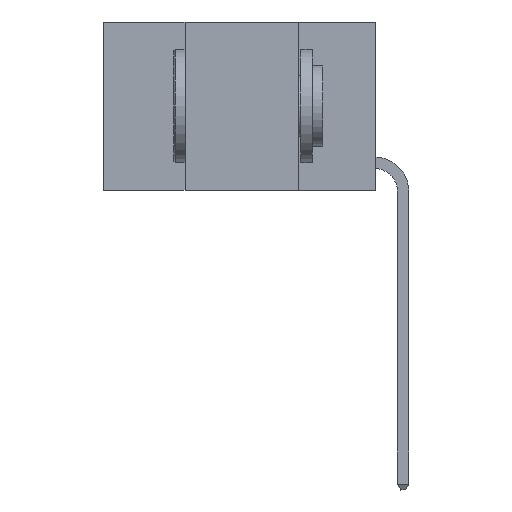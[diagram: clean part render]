
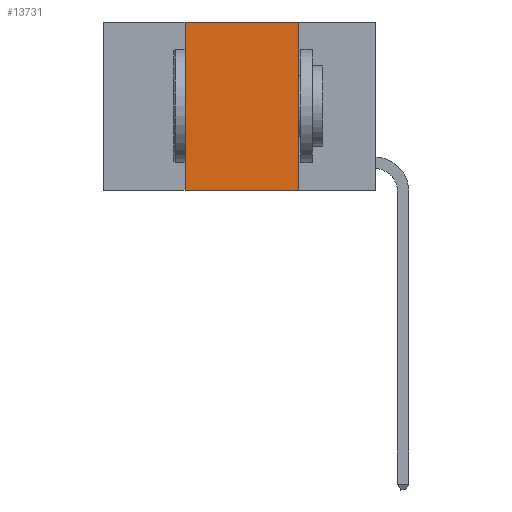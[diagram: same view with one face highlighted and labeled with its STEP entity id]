
A CAD part, left-side view. The second image highlights one B-rep face of the part: STEP entity #13731.
In plain terms, the highlighted planar face has unit normal (-1, 0, 0).
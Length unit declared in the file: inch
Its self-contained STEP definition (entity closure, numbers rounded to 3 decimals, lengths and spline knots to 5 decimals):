
#467 = VERTEX_POINT ( 'NONE', #2920 ) ;
#873 = VECTOR ( 'NONE', #13140, 39.37008 ) ;
#2773 = VERTEX_POINT ( 'NONE', #14449 ) ;
#2920 = CARTESIAN_POINT ( 'NONE',  ( 0., 0.17, 0. ) ) ;
#3199 = EDGE_CURVE ( 'NONE', #2773, #18432, #14423, .T. ) ;
#5081 = ORIENTED_EDGE ( 'NONE', *, *, #13745, .F. ) ;
#6326 = CARTESIAN_POINT ( 'NONE',  ( 0., 0.6, 0. ) ) ;
#6336 = VERTEX_POINT ( 'NONE', #13965 ) ;
#6507 = CARTESIAN_POINT ( 'NONE',  ( 0., 0.42, 0. ) ) ;
#7191 = EDGE_CURVE ( 'NONE', #467, #18432, #13002, .T. ) ;
#8119 = FACE_OUTER_BOUND ( 'NONE', #16934, .T. ) ;
#8319 = VECTOR ( 'NONE', #13219, 39.37008 ) ;
#9045 = CARTESIAN_POINT ( 'NONE',  ( 0., 0.17, -0.37 ) ) ;
#9633 = DIRECTION ( 'NONE',  ( 0., -1., 0. ) ) ;
#9694 = DIRECTION ( 'NONE',  ( 1., 0., 0. ) ) ;
#9911 = EDGE_CURVE ( 'NONE', #2773, #6336, #11960, .T. ) ;
#10307 = VECTOR ( 'NONE', #18775, 39.37008 ) ;
#11960 = LINE ( 'NONE', #6507, #10307 ) ;
#13002 = LINE ( 'NONE', #13103, #8319 ) ;
#13103 = CARTESIAN_POINT ( 'NONE',  ( 0., 0.17, 0. ) ) ;
#13140 = DIRECTION ( 'NONE',  ( 0., -1., 0. ) ) ;
#13219 = DIRECTION ( 'NONE',  ( 0., 0., -1. ) ) ;
#13731 = ADVANCED_FACE ( 'NONE', ( #8119 ), #19836, .F. ) ;
#13745 = EDGE_CURVE ( 'NONE', #6336, #467, #18281, .T. ) ;
#13965 = CARTESIAN_POINT ( 'NONE',  ( 0., 0.42, 0. ) ) ;
#14423 = LINE ( 'NONE', #19679, #17521 ) ;
#14449 = CARTESIAN_POINT ( 'NONE',  ( 0., 0.42, -0.37 ) ) ;
#14853 = ORIENTED_EDGE ( 'NONE', *, *, #3199, .T. ) ;
#15853 = DIRECTION ( 'NONE',  ( 0., 0., -1. ) ) ;
#15963 = CARTESIAN_POINT ( 'NONE',  ( 0., 0.6, 0. ) ) ;
#16270 = ORIENTED_EDGE ( 'NONE', *, *, #9911, .F. ) ;
#16934 = EDGE_LOOP ( 'NONE', ( #21016, #5081, #16270, #14853 ) ) ;
#17521 = VECTOR ( 'NONE', #9633, 39.37008 ) ;
#18281 = LINE ( 'NONE', #15963, #873 ) ;
#18432 = VERTEX_POINT ( 'NONE', #9045 ) ;
#18775 = DIRECTION ( 'NONE',  ( 0., 0., 1. ) ) ;
#19679 = CARTESIAN_POINT ( 'NONE',  ( 0., 0.6, -0.37 ) ) ;
#19836 = PLANE ( 'NONE',  #20413 ) ;
#20413 = AXIS2_PLACEMENT_3D ( 'NONE', #6326, #9694, #15853 ) ;
#21016 = ORIENTED_EDGE ( 'NONE', *, *, #7191, .F. ) ;
